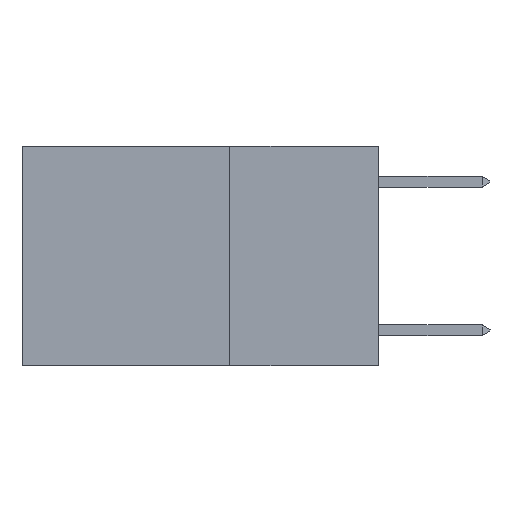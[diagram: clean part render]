
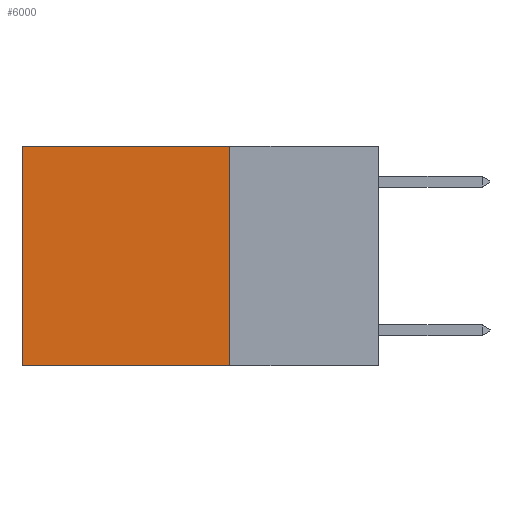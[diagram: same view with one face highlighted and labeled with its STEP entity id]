
A CAD part, left-side view. The second image highlights one B-rep face of the part: STEP entity #6000.
In plain terms, the highlighted planar face has unit normal (-1, 0, 0).
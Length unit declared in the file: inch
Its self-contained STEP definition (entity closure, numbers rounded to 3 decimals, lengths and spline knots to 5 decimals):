
#97 = FACE_OUTER_BOUND ( 'NONE', #6535, .T. ) ;
#546 = CARTESIAN_POINT ( 'NONE',  ( 0.2625, 0.25, 0. ) ) ;
#1582 = ORIENTED_EDGE ( 'NONE', *, *, #1838, .F. ) ;
#1838 = EDGE_CURVE ( 'NONE', #2953, #9039, #4641, .T. ) ;
#2479 = PLANE ( 'NONE',  #6042 ) ;
#2953 = VERTEX_POINT ( 'NONE', #11795 ) ;
#3633 = CARTESIAN_POINT ( 'NONE',  ( 0.2625, 0.25, 0. ) ) ;
#3636 = LINE ( 'NONE', #3633, #11246 ) ;
#4127 = CARTESIAN_POINT ( 'NONE',  ( 0.2625, 0.6, 0. ) ) ;
#4130 = VERTEX_POINT ( 'NONE', #546 ) ;
#4456 = DIRECTION ( 'NONE',  ( 0., 0., -1. ) ) ;
#4641 = LINE ( 'NONE', #9927, #6024 ) ;
#5029 = CARTESIAN_POINT ( 'NONE',  ( 0.2625, 0.6, -0.37 ) ) ;
#5417 = CARTESIAN_POINT ( 'NONE',  ( 0.2625, 0.25, 0. ) ) ;
#5449 = ORIENTED_EDGE ( 'NONE', *, *, #10074, .F. ) ;
#6000 = ADVANCED_FACE ( 'NONE', ( #97 ), #2479, .F. ) ;
#6024 = VECTOR ( 'NONE', #6385, 39.37008 ) ;
#6042 = AXIS2_PLACEMENT_3D ( 'NONE', #5417, #6510, #4456 ) ;
#6385 = DIRECTION ( 'NONE',  ( 0., 1., 0. ) ) ;
#6394 = DIRECTION ( 'NONE',  ( 0., 0., -1. ) ) ;
#6510 = DIRECTION ( 'NONE',  ( 1., 0., 0. ) ) ;
#6535 = EDGE_LOOP ( 'NONE', ( #9770, #1582, #5449, #7653 ) ) ;
#7061 = VECTOR ( 'NONE', #11354, 39.37008 ) ;
#7174 = EDGE_CURVE ( 'NONE', #4130, #11237, #3636, .T. ) ;
#7653 = ORIENTED_EDGE ( 'NONE', *, *, #7174, .T. ) ;
#7812 = DIRECTION ( 'NONE',  ( 0., 1., 0. ) ) ;
#9039 = VERTEX_POINT ( 'NONE', #5029 ) ;
#9770 = ORIENTED_EDGE ( 'NONE', *, *, #10371, .T. ) ;
#9927 = CARTESIAN_POINT ( 'NONE',  ( 0.2625, 0.25, -0.37 ) ) ;
#10074 = EDGE_CURVE ( 'NONE', #4130, #2953, #12266, .T. ) ;
#10371 = EDGE_CURVE ( 'NONE', #11237, #9039, #11928, .T. ) ;
#10384 = CARTESIAN_POINT ( 'NONE',  ( 0.2625, 0.25, 0. ) ) ;
#10866 = VECTOR ( 'NONE', #6394, 39.37008 ) ;
#11237 = VERTEX_POINT ( 'NONE', #4127 ) ;
#11246 = VECTOR ( 'NONE', #7812, 39.37008 ) ;
#11354 = DIRECTION ( 'NONE',  ( 0., 0., -1. ) ) ;
#11535 = CARTESIAN_POINT ( 'NONE',  ( 0.2625, 0.6, 0. ) ) ;
#11795 = CARTESIAN_POINT ( 'NONE',  ( 0.2625, 0.25, -0.37 ) ) ;
#11928 = LINE ( 'NONE', #11535, #10866 ) ;
#12266 = LINE ( 'NONE', #10384, #7061 ) ;
